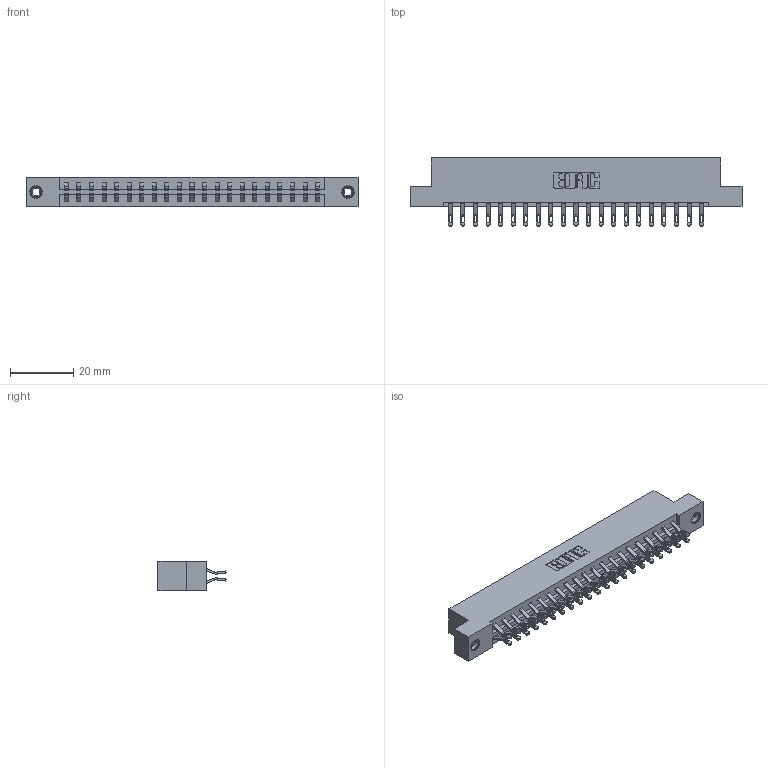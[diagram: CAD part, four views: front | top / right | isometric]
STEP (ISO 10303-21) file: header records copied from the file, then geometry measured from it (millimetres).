
FILE_DESCRIPTION (( 'STEP AP203' ), '1' );
FILE_NAME ('333-042-555-207.STEP', '2018-08-03T19:24:35', ( '' ), ( '' ), 'SwSTEP 2.0', 'SolidWorks 2016', '' );
FILE_SCHEMA (( 'CONFIG_CONTROL_DESIGN' ));
Length unit declared in the file: inch
Products named in the file (4): 333 Part_Flush - .156 Dia - TI; 345-292-001_555 Tail; 345-250-001_345-250-005-103; 333-042-555-207
Assembly tree (45 placements, depth 2):
  333-042-555-207
    333 Part_Flush - .156 Dia - TI
    345-292-001_555 Tail  x42
    345-250-001_345-250-005-103  x2
Bounding box: 104.75 x 21.47 x 9.4 mm (x, y, z)
Volume: 10606.3 mm3; surface area: 12803.3 mm2
Topology: 45 solids, 45 shells, 2610 faces, 8133 edges, 5414 vertices
Faces by surface type: plane 1530, cylinder 1064, cone 12, torus 4
Entity records: 17738 total; most frequent: CARTESIAN_POINT 2983, ORIENTED_EDGE 2882, DIRECTION 2587, EDGE_CURVE 1441, LINE 1273, VECTOR 1273, VERTEX_POINT 956, AXIS2_PLACEMENT_3D 657
